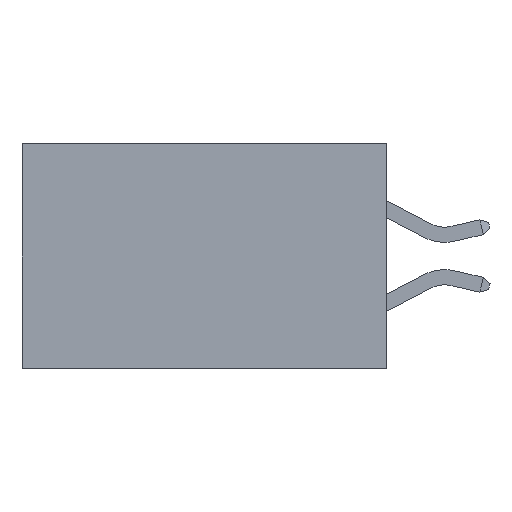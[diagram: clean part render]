
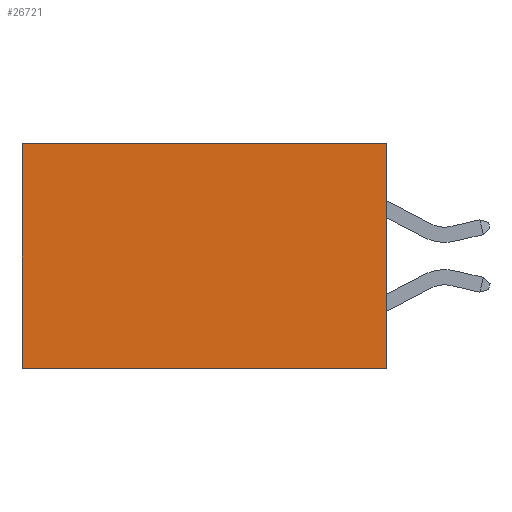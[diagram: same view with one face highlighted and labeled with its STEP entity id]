
A CAD part, left-side view. The second image highlights one B-rep face of the part: STEP entity #26721.
In plain terms, the highlighted planar face has unit normal (-1, 0, 0).
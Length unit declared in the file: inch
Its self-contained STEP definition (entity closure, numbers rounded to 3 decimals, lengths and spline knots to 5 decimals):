
#199 = EDGE_CURVE ( 'NONE', #14794, #9262, #9065, .T. ) ;
#1111 = DIRECTION ( 'NONE',  ( 0., 1., 0. ) ) ;
#2637 = VECTOR ( 'NONE', #1111, 39.37008 ) ;
#2853 = DIRECTION ( 'NONE',  ( 0., 1., 0. ) ) ;
#3515 = ORIENTED_EDGE ( 'NONE', *, *, #22956, .F. ) ;
#3765 = CARTESIAN_POINT ( 'NONE',  ( 0.2615, 0., 0. ) ) ;
#3798 = ORIENTED_EDGE ( 'NONE', *, *, #19605, .T. ) ;
#4613 = EDGE_LOOP ( 'NONE', ( #3798, #13933, #3515, #9355 ) ) ;
#5130 = PLANE ( 'NONE',  #27238 ) ;
#5164 = VECTOR ( 'NONE', #8685, 39.37008 ) ;
#6497 = CARTESIAN_POINT ( 'NONE',  ( 0.2615, 0., -0.37 ) ) ;
#6845 = CARTESIAN_POINT ( 'NONE',  ( 0.2615, 0.6, 0. ) ) ;
#7045 = VERTEX_POINT ( 'NONE', #14760 ) ;
#8685 = DIRECTION ( 'NONE',  ( 0., 0., -1. ) ) ;
#8770 = VECTOR ( 'NONE', #2853, 39.37008 ) ;
#9065 = LINE ( 'NONE', #3765, #2637 ) ;
#9262 = VERTEX_POINT ( 'NONE', #6845 ) ;
#9355 = ORIENTED_EDGE ( 'NONE', *, *, #199, .T. ) ;
#9783 = CARTESIAN_POINT ( 'NONE',  ( 0.2615, 0., 0. ) ) ;
#10506 = FACE_OUTER_BOUND ( 'NONE', #4613, .T. ) ;
#11113 = VERTEX_POINT ( 'NONE', #25413 ) ;
#11556 = LINE ( 'NONE', #13008, #5164 ) ;
#11619 = DIRECTION ( 'NONE',  ( 1., 0., 0. ) ) ;
#12046 = LINE ( 'NONE', #6497, #22631 ) ;
#13008 = CARTESIAN_POINT ( 'NONE',  ( 0.2615, 0.6, -0.37 ) ) ;
#13707 = CARTESIAN_POINT ( 'NONE',  ( 0.2615, 0., -0.37 ) ) ;
#13933 = ORIENTED_EDGE ( 'NONE', *, *, #15280, .F. ) ;
#14491 = LINE ( 'NONE', #13707, #8770 ) ;
#14760 = CARTESIAN_POINT ( 'NONE',  ( 0.2615, 0., -0.37 ) ) ;
#14794 = VERTEX_POINT ( 'NONE', #9783 ) ;
#15280 = EDGE_CURVE ( 'NONE', #7045, #11113, #14491, .T. ) ;
#19605 = EDGE_CURVE ( 'NONE', #9262, #11113, #11556, .T. ) ;
#22631 = VECTOR ( 'NONE', #23499, 39.37008 ) ;
#22956 = EDGE_CURVE ( 'NONE', #14794, #7045, #12046, .T. ) ;
#23499 = DIRECTION ( 'NONE',  ( 0., 0., -1. ) ) ;
#24288 = CARTESIAN_POINT ( 'NONE',  ( 0.2615, 0., -0.37 ) ) ;
#25413 = CARTESIAN_POINT ( 'NONE',  ( 0.2615, 0.6, -0.37 ) ) ;
#26384 = DIRECTION ( 'NONE',  ( 0., 0., -1. ) ) ;
#26721 = ADVANCED_FACE ( 'NONE', ( #10506 ), #5130, .F. ) ;
#27238 = AXIS2_PLACEMENT_3D ( 'NONE', #24288, #11619, #26384 ) ;
